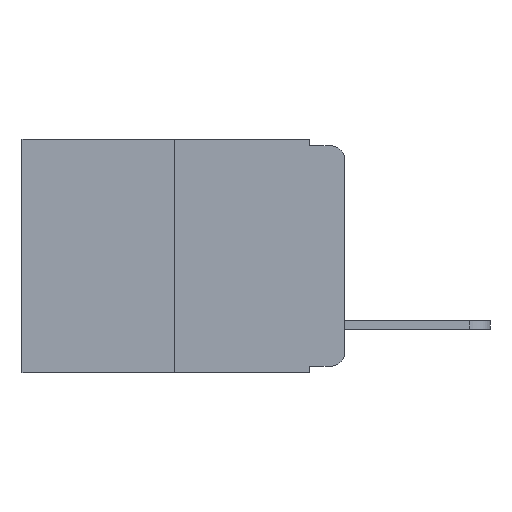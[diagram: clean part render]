
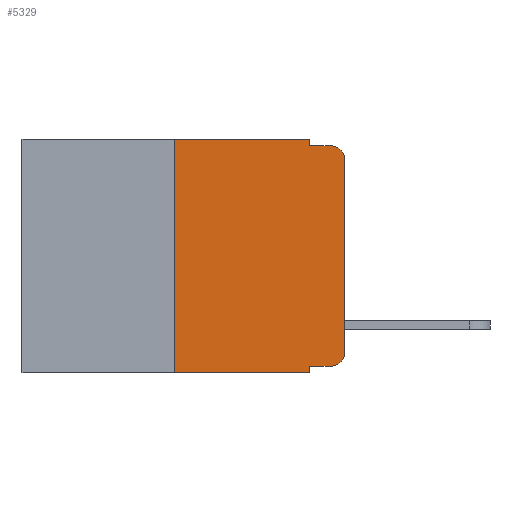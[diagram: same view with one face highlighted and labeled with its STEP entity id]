
A CAD part, left-side view. The second image highlights one B-rep face of the part: STEP entity #5329.
In plain terms, the highlighted planar face has unit normal (-1, 0, 0).
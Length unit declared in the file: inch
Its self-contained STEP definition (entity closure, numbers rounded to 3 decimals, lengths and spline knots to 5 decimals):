
#31 = ORIENTED_EDGE ( 'NONE', *, *, #8293, .F. ) ;
#60 = ORIENTED_EDGE ( 'NONE', *, *, #8197, .T. ) ;
#81 = DIRECTION ( 'NONE',  ( 0., -1., 0. ) ) ;
#1082 = DIRECTION ( 'NONE',  ( 0., 0., 1. ) ) ;
#1108 = CARTESIAN_POINT ( 'NONE',  ( 0., 0., 0. ) ) ;
#1194 = VECTOR ( 'NONE', #81, 39.37008 ) ;
#1196 = CARTESIAN_POINT ( 'NONE',  ( 0., 0.25, 0. ) ) ;
#1277 = VECTOR ( 'NONE', #1082, 39.37008 ) ;
#1316 = LINE ( 'NONE', #6376, #1194 ) ;
#1383 = CARTESIAN_POINT ( 'NONE',  ( 0., 0.051, -0.01 ) ) ;
#1740 = AXIS2_PLACEMENT_3D ( 'NONE', #10910, #10673, #10993 ) ;
#2058 = EDGE_CURVE ( 'NONE', #3486, #10646, #1316, .T. ) ;
#2191 = VERTEX_POINT ( 'NONE', #9270 ) ;
#2478 = CARTESIAN_POINT ( 'NONE',  ( 0., 0., -0.03 ) ) ;
#2492 = CARTESIAN_POINT ( 'NONE',  ( 0., 0.051, 0. ) ) ;
#2524 = VECTOR ( 'NONE', #7471, 39.37008 ) ;
#2740 = CIRCLE ( 'NONE', #3510, 0.02 ) ;
#2757 = LINE ( 'NONE', #1108, #1277 ) ;
#2911 = VECTOR ( 'NONE', #9071, 39.37008 ) ;
#3413 = DIRECTION ( 'NONE',  ( 0., -1., 0. ) ) ;
#3486 = VERTEX_POINT ( 'NONE', #1196 ) ;
#3510 = AXIS2_PLACEMENT_3D ( 'NONE', #10327, #10315, #8750 ) ;
#3615 = VERTEX_POINT ( 'NONE', #7825 ) ;
#3815 = VECTOR ( 'NONE', #3413, 39.37008 ) ;
#4488 = EDGE_CURVE ( 'NONE', #4586, #2191, #8436, .T. ) ;
#4586 = VERTEX_POINT ( 'NONE', #2478 ) ;
#4747 = LINE ( 'NONE', #9351, #6661 ) ;
#5099 = VERTEX_POINT ( 'NONE', #7786 ) ;
#5329 = ADVANCED_FACE ( 'NONE', ( #8121 ), #10935, .F. ) ;
#5593 = LINE ( 'NONE', #9104, #2911 ) ;
#5953 = EDGE_CURVE ( 'NONE', #5099, #4586, #2757, .T. ) ;
#6229 = LINE ( 'NONE', #12179, #8391 ) ;
#6276 = DIRECTION ( 'NONE',  ( 0., 0., 1. ) ) ;
#6357 = LINE ( 'NONE', #1383, #3815 ) ;
#6376 = CARTESIAN_POINT ( 'NONE',  ( 0., 0.473, 0. ) ) ;
#6427 = ORIENTED_EDGE ( 'NONE', *, *, #8011, .T. ) ;
#6428 = DIRECTION ( 'NONE',  ( 0., 0., -1. ) ) ;
#6435 = DIRECTION ( 'NONE',  ( -1., 0., 0. ) ) ;
#6451 = CARTESIAN_POINT ( 'NONE',  ( 0., 0.02, -0.03 ) ) ;
#6661 = VECTOR ( 'NONE', #8653, 39.37008 ) ;
#7252 = VERTEX_POINT ( 'NONE', #10069 ) ;
#7441 = CARTESIAN_POINT ( 'NONE',  ( 0., 0.051, 0. ) ) ;
#7471 = DIRECTION ( 'NONE',  ( 0., 0., -1. ) ) ;
#7680 = EDGE_CURVE ( 'NONE', #7252, #11388, #6229, .T. ) ;
#7786 = CARTESIAN_POINT ( 'NONE',  ( 0., 0., -0.313 ) ) ;
#7825 = CARTESIAN_POINT ( 'NONE',  ( 0., 0.051, -0.333 ) ) ;
#8011 = EDGE_CURVE ( 'NONE', #11341, #5099, #2740, .T. ) ;
#8121 = FACE_OUTER_BOUND ( 'NONE', #10818, .T. ) ;
#8197 = EDGE_CURVE ( 'NONE', #3615, #11341, #5593, .T. ) ;
#8240 = VECTOR ( 'NONE', #6276, 39.37008 ) ;
#8293 = EDGE_CURVE ( 'NONE', #3615, #11388, #4747, .T. ) ;
#8391 = VECTOR ( 'NONE', #8870, 39.37008 ) ;
#8392 = EDGE_CURVE ( 'NONE', #7252, #3486, #10441, .T. ) ;
#8436 = CIRCLE ( 'NONE', #9970, 0.02 ) ;
#8653 = DIRECTION ( 'NONE',  ( 0., 0., -1. ) ) ;
#8750 = DIRECTION ( 'NONE',  ( 0., 0., -1. ) ) ;
#8774 = EDGE_CURVE ( 'NONE', #10646, #10384, #10031, .T. ) ;
#8870 = DIRECTION ( 'NONE',  ( 0., -1., 0. ) ) ;
#9016 = EDGE_CURVE ( 'NONE', #10384, #2191, #6357, .T. ) ;
#9071 = DIRECTION ( 'NONE',  ( 0., -1., 0. ) ) ;
#9104 = CARTESIAN_POINT ( 'NONE',  ( 0., 0.051, -0.333 ) ) ;
#9194 = CARTESIAN_POINT ( 'NONE',  ( 0., 0.25, 0. ) ) ;
#9270 = CARTESIAN_POINT ( 'NONE',  ( 0., 0.02, -0.01 ) ) ;
#9351 = CARTESIAN_POINT ( 'NONE',  ( 0., 0.051, 0. ) ) ;
#9970 = AXIS2_PLACEMENT_3D ( 'NONE', #6451, #6435, #6428 ) ;
#10031 = LINE ( 'NONE', #7441, #2524 ) ;
#10069 = CARTESIAN_POINT ( 'NONE',  ( 0., 0.25, -0.343 ) ) ;
#10297 = ORIENTED_EDGE ( 'NONE', *, *, #5953, .T. ) ;
#10315 = DIRECTION ( 'NONE',  ( -1., 0., 0. ) ) ;
#10327 = CARTESIAN_POINT ( 'NONE',  ( 0., 0.02, -0.313 ) ) ;
#10384 = VERTEX_POINT ( 'NONE', #10547 ) ;
#10441 = LINE ( 'NONE', #9194, #8240 ) ;
#10500 = ORIENTED_EDGE ( 'NONE', *, *, #4488, .T. ) ;
#10547 = CARTESIAN_POINT ( 'NONE',  ( 0., 0.051, -0.01 ) ) ;
#10646 = VERTEX_POINT ( 'NONE', #2492 ) ;
#10673 = DIRECTION ( 'NONE',  ( 1., 0., 0. ) ) ;
#10690 = ORIENTED_EDGE ( 'NONE', *, *, #9016, .F. ) ;
#10765 = ORIENTED_EDGE ( 'NONE', *, *, #8774, .F. ) ;
#10805 = ORIENTED_EDGE ( 'NONE', *, *, #2058, .F. ) ;
#10818 = EDGE_LOOP ( 'NONE', ( #10297, #10500, #10690, #10765, #10805, #10929, #12263, #31, #60, #6427 ) ) ;
#10864 = CARTESIAN_POINT ( 'NONE',  ( 0., 0.051, -0.343 ) ) ;
#10910 = CARTESIAN_POINT ( 'NONE',  ( 0., 0.473, 0. ) ) ;
#10929 = ORIENTED_EDGE ( 'NONE', *, *, #8392, .F. ) ;
#10935 = PLANE ( 'NONE',  #1740 ) ;
#10993 = DIRECTION ( 'NONE',  ( 0., 0., -1. ) ) ;
#11341 = VERTEX_POINT ( 'NONE', #11692 ) ;
#11388 = VERTEX_POINT ( 'NONE', #10864 ) ;
#11692 = CARTESIAN_POINT ( 'NONE',  ( 0., 0.02, -0.333 ) ) ;
#12179 = CARTESIAN_POINT ( 'NONE',  ( 0., 0.473, -0.343 ) ) ;
#12263 = ORIENTED_EDGE ( 'NONE', *, *, #7680, .T. ) ;
